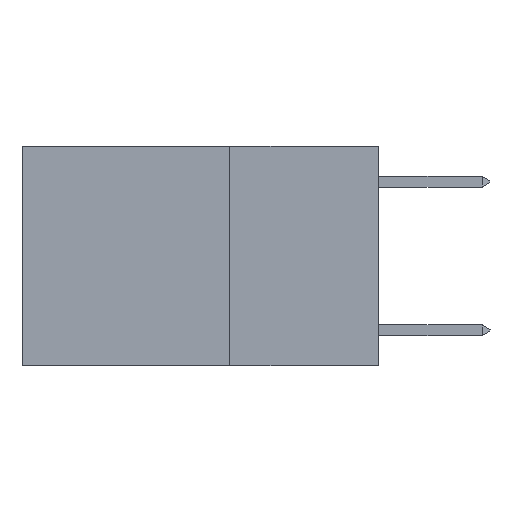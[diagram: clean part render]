
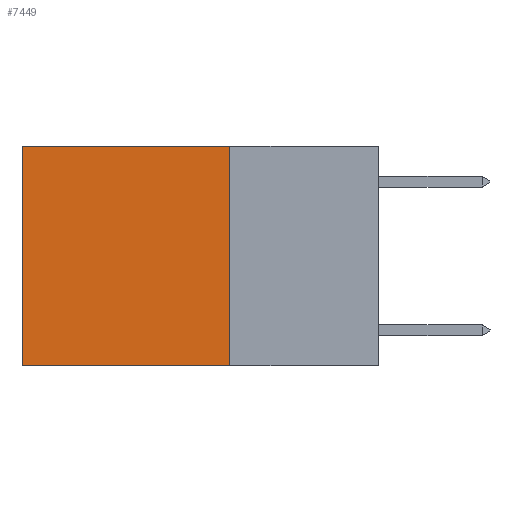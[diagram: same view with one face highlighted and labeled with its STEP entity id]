
A CAD part, left-side view. The second image highlights one B-rep face of the part: STEP entity #7449.
In plain terms, the highlighted planar face has unit normal (-1, 0, 0).
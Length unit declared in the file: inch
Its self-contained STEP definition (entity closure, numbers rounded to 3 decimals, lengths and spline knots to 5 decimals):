
#302 = VECTOR ( 'NONE', #4654, 39.37008 ) ;
#473 = CARTESIAN_POINT ( 'NONE',  ( 0.2625, 0.6, 0. ) ) ;
#580 = EDGE_CURVE ( 'NONE', #2129, #2336, #7620, .T. ) ;
#1703 = VECTOR ( 'NONE', #10103, 39.37008 ) ;
#1713 = ORIENTED_EDGE ( 'NONE', *, *, #7566, .F. ) ;
#1915 = DIRECTION ( 'NONE',  ( 0., 0., -1. ) ) ;
#2056 = CARTESIAN_POINT ( 'NONE',  ( 0.2625, 0.25, 0. ) ) ;
#2129 = VERTEX_POINT ( 'NONE', #9877 ) ;
#2213 = ORIENTED_EDGE ( 'NONE', *, *, #580, .F. ) ;
#2262 = CARTESIAN_POINT ( 'NONE',  ( 0.2625, 0.25, 0. ) ) ;
#2336 = VERTEX_POINT ( 'NONE', #2538 ) ;
#2416 = VECTOR ( 'NONE', #8229, 39.37008 ) ;
#2538 = CARTESIAN_POINT ( 'NONE',  ( 0.2625, 0.6, -0.37 ) ) ;
#2572 = DIRECTION ( 'NONE',  ( 0., 1., 0. ) ) ;
#3058 = LINE ( 'NONE', #4956, #2416 ) ;
#3143 = VERTEX_POINT ( 'NONE', #473 ) ;
#3996 = EDGE_CURVE ( 'NONE', #8367, #3143, #10179, .T. ) ;
#4019 = EDGE_LOOP ( 'NONE', ( #5223, #2213, #1713, #8570 ) ) ;
#4369 = DIRECTION ( 'NONE',  ( 1., 0., 0. ) ) ;
#4654 = DIRECTION ( 'NONE',  ( 0., 0., -1. ) ) ;
#4956 = CARTESIAN_POINT ( 'NONE',  ( 0.2625, 0.6, 0. ) ) ;
#5223 = ORIENTED_EDGE ( 'NONE', *, *, #8623, .T. ) ;
#5615 = VECTOR ( 'NONE', #2572, 39.37008 ) ;
#6535 = CARTESIAN_POINT ( 'NONE',  ( 0.2625, 0.25, -0.37 ) ) ;
#6998 = LINE ( 'NONE', #10260, #302 ) ;
#7390 = FACE_OUTER_BOUND ( 'NONE', #4019, .T. ) ;
#7449 = ADVANCED_FACE ( 'NONE', ( #7390 ), #8460, .F. ) ;
#7566 = EDGE_CURVE ( 'NONE', #8367, #2129, #6998, .T. ) ;
#7620 = LINE ( 'NONE', #6535, #5615 ) ;
#8229 = DIRECTION ( 'NONE',  ( 0., 0., -1. ) ) ;
#8367 = VERTEX_POINT ( 'NONE', #2262 ) ;
#8460 = PLANE ( 'NONE',  #9379 ) ;
#8570 = ORIENTED_EDGE ( 'NONE', *, *, #3996, .T. ) ;
#8623 = EDGE_CURVE ( 'NONE', #3143, #2336, #3058, .T. ) ;
#9379 = AXIS2_PLACEMENT_3D ( 'NONE', #10108, #4369, #1915 ) ;
#9877 = CARTESIAN_POINT ( 'NONE',  ( 0.2625, 0.25, -0.37 ) ) ;
#10103 = DIRECTION ( 'NONE',  ( 0., 1., 0. ) ) ;
#10108 = CARTESIAN_POINT ( 'NONE',  ( 0.2625, 0.25, 0. ) ) ;
#10179 = LINE ( 'NONE', #2056, #1703 ) ;
#10260 = CARTESIAN_POINT ( 'NONE',  ( 0.2625, 0.25, 0. ) ) ;
